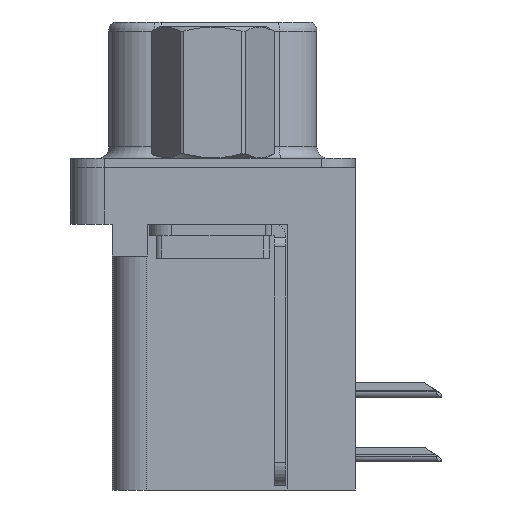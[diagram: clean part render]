
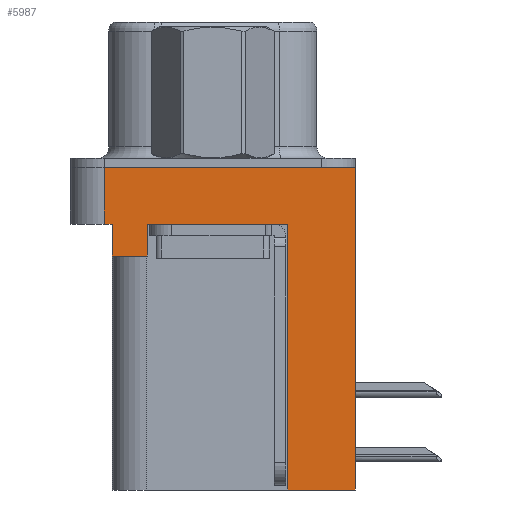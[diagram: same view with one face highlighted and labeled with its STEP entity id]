
A CAD part, left-side view. The second image highlights one B-rep face of the part: STEP entity #5987.
In plain terms, the highlighted planar face has unit normal (-1, 0, 0).
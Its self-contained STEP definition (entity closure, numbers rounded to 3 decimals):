
#84 = DIRECTION ( 'NONE',  ( 0., 0., 1. ) ) ;
#88 = ORIENTED_EDGE ( 'NONE', *, *, #12858, .F. ) ;
#361 = VERTEX_POINT ( 'NONE', #24260 ) ;
#415 = CARTESIAN_POINT ( 'NONE',  ( -3., 4.775, -2.5 ) ) ;
#426 = ORIENTED_EDGE ( 'NONE', *, *, #24535, .F. ) ;
#706 = DIRECTION ( 'NONE',  ( 0., -1., 0. ) ) ;
#1264 = CARTESIAN_POINT ( 'NONE',  ( -3., 4.425, -3.9 ) ) ;
#1284 = EDGE_CURVE ( 'NONE', #25017, #20487, #6913, .T. ) ;
#1308 = CARTESIAN_POINT ( 'NONE',  ( -3., -6.275, -2.5 ) ) ;
#1523 = LINE ( 'NONE', #1264, #20211 ) ;
#1739 = LINE ( 'NONE', #10208, #10393 ) ;
#2258 = ORIENTED_EDGE ( 'NONE', *, *, #21487, .F. ) ;
#2426 = VECTOR ( 'NONE', #9782, 1000. ) ;
#2796 = EDGE_CURVE ( 'NONE', #361, #14060, #22201, .T. ) ;
#2977 = ORIENTED_EDGE ( 'NONE', *, *, #24977, .T. ) ;
#3188 = CARTESIAN_POINT ( 'NONE',  ( -3., -6.275, 0. ) ) ;
#3341 = DIRECTION ( 'NONE',  ( 0., 0., 1. ) ) ;
#4142 = EDGE_CURVE ( 'NONE', #9343, #14060, #11324, .T. ) ;
#4636 = LINE ( 'NONE', #4778, #15065 ) ;
#4778 = CARTESIAN_POINT ( 'NONE',  ( -3., 4.775, -2.5 ) ) ;
#5477 = CARTESIAN_POINT ( 'NONE',  ( -3., 2.895, -2.5 ) ) ;
#5959 = ORIENTED_EDGE ( 'NONE', *, *, #15979, .T. ) ;
#5987 = ADVANCED_FACE ( 'NONE', ( #12557 ), #6619, .T. ) ;
#6353 = CARTESIAN_POINT ( 'NONE',  ( -3., 2.895, -3.9 ) ) ;
#6619 = PLANE ( 'NONE',  #16424 ) ;
#6762 = VECTOR ( 'NONE', #15349, 1000. ) ;
#6913 = LINE ( 'NONE', #13002, #6762 ) ;
#9074 = EDGE_CURVE ( 'NONE', #24121, #11477, #15072, .T. ) ;
#9088 = ORIENTED_EDGE ( 'NONE', *, *, #9074, .F. ) ;
#9185 = VECTOR ( 'NONE', #706, 1000. ) ;
#9343 = VERTEX_POINT ( 'NONE', #24210 ) ;
#9782 = DIRECTION ( 'NONE',  ( 0., -1., 0. ) ) ;
#10208 = CARTESIAN_POINT ( 'NONE',  ( -3., -3.295, -14.2 ) ) ;
#10393 = VECTOR ( 'NONE', #18654, 1000. ) ;
#11324 = LINE ( 'NONE', #24104, #18343 ) ;
#11327 = CARTESIAN_POINT ( 'NONE',  ( -3., -6.275, 0. ) ) ;
#11477 = VERTEX_POINT ( 'NONE', #14835 ) ;
#12557 = FACE_OUTER_BOUND ( 'NONE', #19419, .T. ) ;
#12858 = EDGE_CURVE ( 'NONE', #11477, #16398, #1523, .T. ) ;
#13002 = CARTESIAN_POINT ( 'NONE',  ( -3., -3.295, -14.2 ) ) ;
#13058 = LINE ( 'NONE', #13339, #9185 ) ;
#13339 = CARTESIAN_POINT ( 'NONE',  ( -3., -6.275, -2.5 ) ) ;
#13770 = CARTESIAN_POINT ( 'NONE',  ( -3., 2.895, -3.9 ) ) ;
#13858 = DIRECTION ( 'NONE',  ( 0., -1., 0. ) ) ;
#13938 = CARTESIAN_POINT ( 'NONE',  ( -3., 4.425, -2.5 ) ) ;
#14060 = VERTEX_POINT ( 'NONE', #11327 ) ;
#14835 = CARTESIAN_POINT ( 'NONE',  ( -3., 4.425, -3.9 ) ) ;
#15065 = VECTOR ( 'NONE', #21559, 1000. ) ;
#15072 = LINE ( 'NONE', #21322, #18737 ) ;
#15349 = DIRECTION ( 'NONE',  ( 0., 0., 1. ) ) ;
#15979 = EDGE_CURVE ( 'NONE', #18969, #20487, #13058, .T. ) ;
#15994 = LINE ( 'NONE', #13770, #24410 ) ;
#16398 = VERTEX_POINT ( 'NONE', #13938 ) ;
#16424 = AXIS2_PLACEMENT_3D ( 'NONE', #17131, #18942, #84 ) ;
#16873 = DIRECTION ( 'NONE',  ( 0., 1., 0. ) ) ;
#16920 = VECTOR ( 'NONE', #13858, 1000. ) ;
#17131 = CARTESIAN_POINT ( 'NONE',  ( -3., -6.275, -2.5 ) ) ;
#17684 = CARTESIAN_POINT ( 'NONE',  ( -3., -3.295, -2.5 ) ) ;
#17796 = DIRECTION ( 'NONE',  ( 0., 0., 1. ) ) ;
#18324 = VERTEX_POINT ( 'NONE', #415 ) ;
#18343 = VECTOR ( 'NONE', #19517, 1000. ) ;
#18654 = DIRECTION ( 'NONE',  ( 0., 1., 0. ) ) ;
#18737 = VECTOR ( 'NONE', #16873, 1000. ) ;
#18942 = DIRECTION ( 'NONE',  ( -1., 0., 0. ) ) ;
#18969 = VERTEX_POINT ( 'NONE', #5477 ) ;
#19419 = EDGE_LOOP ( 'NONE', ( #22322, #2258, #2977, #88, #9088, #21709, #5959, #25359, #426, #24071 ) ) ;
#19517 = DIRECTION ( 'NONE',  ( 0., 0., 1. ) ) ;
#20211 = VECTOR ( 'NONE', #3341, 1000. ) ;
#20487 = VERTEX_POINT ( 'NONE', #17684 ) ;
#21322 = CARTESIAN_POINT ( 'NONE',  ( -3., 4.425, -3.9 ) ) ;
#21487 = EDGE_CURVE ( 'NONE', #18324, #361, #4636, .T. ) ;
#21559 = DIRECTION ( 'NONE',  ( 0., 0., 1. ) ) ;
#21625 = EDGE_CURVE ( 'NONE', #24121, #18969, #15994, .T. ) ;
#21709 = ORIENTED_EDGE ( 'NONE', *, *, #21625, .T. ) ;
#22201 = LINE ( 'NONE', #3188, #16920 ) ;
#22322 = ORIENTED_EDGE ( 'NONE', *, *, #2796, .F. ) ;
#22532 = CARTESIAN_POINT ( 'NONE',  ( -3., -3.295, -14.2 ) ) ;
#24071 = ORIENTED_EDGE ( 'NONE', *, *, #4142, .T. ) ;
#24104 = CARTESIAN_POINT ( 'NONE',  ( -3., -6.275, -2.5 ) ) ;
#24121 = VERTEX_POINT ( 'NONE', #6353 ) ;
#24210 = CARTESIAN_POINT ( 'NONE',  ( -3., -6.275, -14.2 ) ) ;
#24260 = CARTESIAN_POINT ( 'NONE',  ( -3., 4.775, 0. ) ) ;
#24410 = VECTOR ( 'NONE', #17796, 1000. ) ;
#24535 = EDGE_CURVE ( 'NONE', #9343, #25017, #1739, .T. ) ;
#24977 = EDGE_CURVE ( 'NONE', #18324, #16398, #26837, .T. ) ;
#25017 = VERTEX_POINT ( 'NONE', #22532 ) ;
#25359 = ORIENTED_EDGE ( 'NONE', *, *, #1284, .F. ) ;
#26837 = LINE ( 'NONE', #1308, #2426 ) ;
